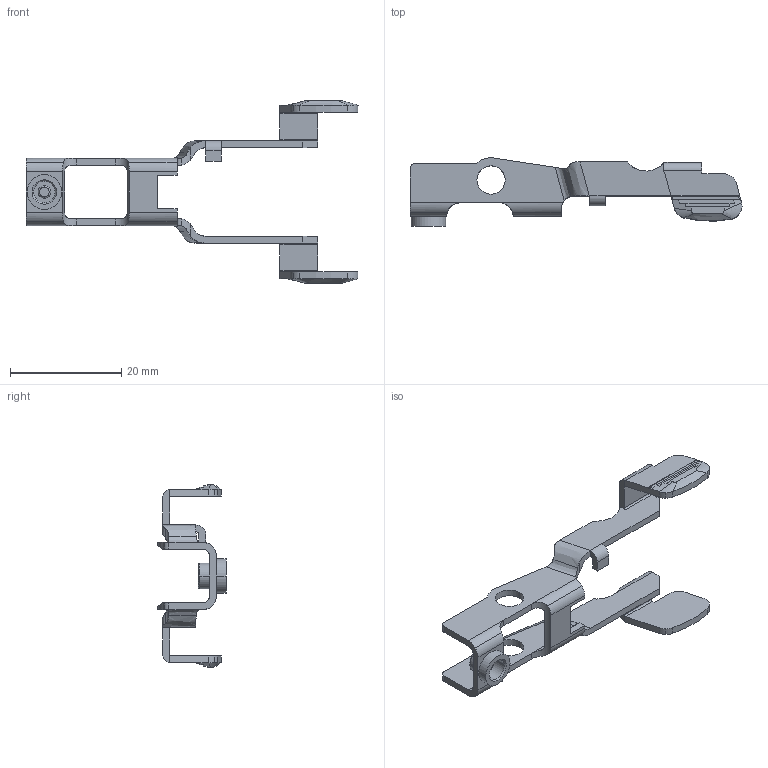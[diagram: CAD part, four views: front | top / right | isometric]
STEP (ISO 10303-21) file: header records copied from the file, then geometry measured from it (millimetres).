
FILE_DESCRIPTION (( 'STEP AP214' ), '1' );
FILE_NAME ('Slide Catch Lever.step', '2014-07-30T19:46:52', ( 'WarFairy' ), ( '' ), 'SwSTEP 2.0', 'SolidWorks 2013', '' );
FILE_SCHEMA (( 'AUTOMOTIVE_DESIGN' ));
Length unit declared in the file: millimetre
Products named in the file (1): Slide Catch Lever
Bounding box: 59.7 x 12.28 x 32.94 mm (x, y, z)
Volume: 1484.1 mm3; surface area: 2845.1 mm2
Topology: 1 solids, 1 shells, 172 faces, 476 edges, 308 vertices
Faces by surface type: plane 76, cylinder 72, bspline 18, torus 4, cone 2
Entity records: 6409 total; most frequent: CARTESIAN_POINT 2130, ORIENTED_EDGE 952, DIRECTION 800, EDGE_CURVE 476, VERTEX_POINT 308, VECTOR 270, LINE 270, AXIS2_PLACEMENT_3D 265
